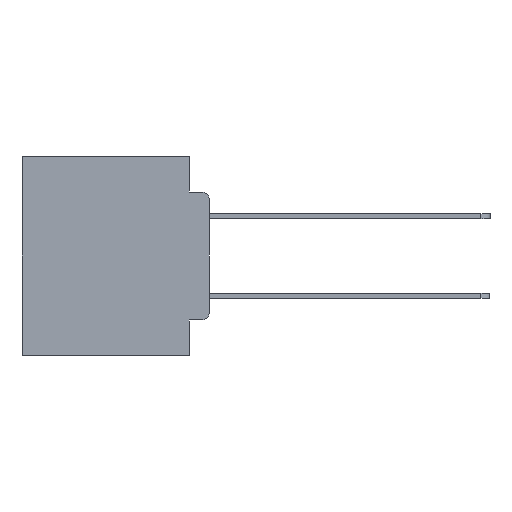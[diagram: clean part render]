
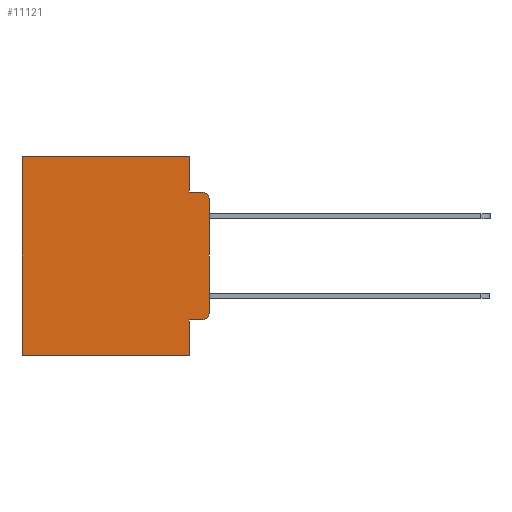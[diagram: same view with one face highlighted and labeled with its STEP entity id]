
A CAD part, left-side view. The second image highlights one B-rep face of the part: STEP entity #11121.
In plain terms, the highlighted planar face has unit normal (-1, 0, 0).
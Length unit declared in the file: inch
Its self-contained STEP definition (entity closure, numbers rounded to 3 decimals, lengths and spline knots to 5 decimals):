
#91 = EDGE_CURVE ( 'NONE', #11731, #8645, #16837, .T. ) ;
#188 = VECTOR ( 'NONE', #9509, 39.37008 ) ;
#833 = ORIENTED_EDGE ( 'NONE', *, *, #21471, .T. ) ;
#1757 = VERTEX_POINT ( 'NONE', #11568 ) ;
#2285 = ORIENTED_EDGE ( 'NONE', *, *, #91, .T. ) ;
#2340 = ORIENTED_EDGE ( 'NONE', *, *, #14090, .T. ) ;
#2466 = VERTEX_POINT ( 'NONE', #26291 ) ;
#2994 = DIRECTION ( 'NONE',  ( 0., -1., 0. ) ) ;
#3147 = VECTOR ( 'NONE', #22898, 39.37008 ) ;
#3359 = EDGE_LOOP ( 'NONE', ( #7922, #2285, #5350, #19987, #15422, #20223, #26096, #23417, #833, #2340 ) ) ;
#3412 = EDGE_CURVE ( 'NONE', #11731, #2466, #8295, .T. ) ;
#3960 = LINE ( 'NONE', #26126, #14698 ) ;
#4420 = VECTOR ( 'NONE', #9666, 39.37008 ) ;
#4872 = CARTESIAN_POINT ( 'NONE',  ( 0.298, 0.02, -0.4115 ) ) ;
#4892 = LINE ( 'NONE', #19153, #26584 ) ;
#5350 = ORIENTED_EDGE ( 'NONE', *, *, #22538, .F. ) ;
#5572 = EDGE_CURVE ( 'NONE', #7478, #25046, #7101, .T. ) ;
#6067 = CARTESIAN_POINT ( 'NONE',  ( 0.298, 0.051, 0. ) ) ;
#6334 = EDGE_CURVE ( 'NONE', #1757, #7478, #11154, .T. ) ;
#6660 = CARTESIAN_POINT ( 'NONE',  ( 0.298, 0.02, -0.1085 ) ) ;
#6828 = EDGE_CURVE ( 'NONE', #21465, #25046, #14746, .T. ) ;
#6844 = CARTESIAN_POINT ( 'NONE',  ( 0.298, 0.051, -0.5 ) ) ;
#7101 = LINE ( 'NONE', #9027, #12868 ) ;
#7158 = DIRECTION ( 'NONE',  ( 0., 0., -1. ) ) ;
#7433 = CARTESIAN_POINT ( 'NONE',  ( 0.298, 0.051, 0. ) ) ;
#7478 = VERTEX_POINT ( 'NONE', #6844 ) ;
#7873 = DIRECTION ( 'NONE',  ( 0., 1., 0. ) ) ;
#7922 = ORIENTED_EDGE ( 'NONE', *, *, #3412, .F. ) ;
#8295 = LINE ( 'NONE', #25210, #13310 ) ;
#8441 = FACE_OUTER_BOUND ( 'NONE', #3359, .T. ) ;
#8645 = VERTEX_POINT ( 'NONE', #16828 ) ;
#9027 = CARTESIAN_POINT ( 'NONE',  ( 0.298, 0., -0.5 ) ) ;
#9509 = DIRECTION ( 'NONE',  ( 0., 0., -1. ) ) ;
#9666 = DIRECTION ( 'NONE',  ( 0., 1., 0. ) ) ;
#10009 = PLANE ( 'NONE',  #25754 ) ;
#10889 = VERTEX_POINT ( 'NONE', #4872 ) ;
#10956 = DIRECTION ( 'NONE',  ( 0., -1., 0. ) ) ;
#11121 = ADVANCED_FACE ( 'NONE', ( #8441 ), #10009, .F. ) ;
#11154 = LINE ( 'NONE', #7433, #188 ) ;
#11568 = CARTESIAN_POINT ( 'NONE',  ( 0.298, 0.051, -0.4115 ) ) ;
#11731 = VERTEX_POINT ( 'NONE', #18914 ) ;
#11760 = VERTEX_POINT ( 'NONE', #13676 ) ;
#11801 = CARTESIAN_POINT ( 'NONE',  ( 0.298, 0., 0. ) ) ;
#12160 = DIRECTION ( 'NONE',  ( 1., 0., 0. ) ) ;
#12718 = VERTEX_POINT ( 'NONE', #18701 ) ;
#12868 = VECTOR ( 'NONE', #7873, 39.37008 ) ;
#12927 = CARTESIAN_POINT ( 'NONE',  ( 0.298, 0.02, -0.3915 ) ) ;
#13310 = VECTOR ( 'NONE', #25956, 39.37008 ) ;
#13333 = AXIS2_PLACEMENT_3D ( 'NONE', #6660, #20187, #7158 ) ;
#13366 = EDGE_CURVE ( 'NONE', #12718, #11760, #14624, .T. ) ;
#13676 = CARTESIAN_POINT ( 'NONE',  ( 0.298, 0.051, -0.0885 ) ) ;
#14090 = EDGE_CURVE ( 'NONE', #10889, #2466, #24205, .T. ) ;
#14343 = DIRECTION ( 'NONE',  ( 0., 0., -1. ) ) ;
#14624 = LINE ( 'NONE', #6067, #3147 ) ;
#14698 = VECTOR ( 'NONE', #2994, 39.37008 ) ;
#14746 = LINE ( 'NONE', #15899, #19580 ) ;
#15022 = DIRECTION ( 'NONE',  ( 0., 0., -1. ) ) ;
#15263 = CARTESIAN_POINT ( 'NONE',  ( 0.298, 0.473, -0.5 ) ) ;
#15422 = ORIENTED_EDGE ( 'NONE', *, *, #19486, .T. ) ;
#15899 = CARTESIAN_POINT ( 'NONE',  ( 0.298, 0.473, 0. ) ) ;
#16828 = CARTESIAN_POINT ( 'NONE',  ( 0.298, 0.02, -0.0885 ) ) ;
#16837 = CIRCLE ( 'NONE', #13333, 0.02 ) ;
#18245 = AXIS2_PLACEMENT_3D ( 'NONE', #12927, #27370, #15022 ) ;
#18701 = CARTESIAN_POINT ( 'NONE',  ( 0.298, 0.051, 0. ) ) ;
#18914 = CARTESIAN_POINT ( 'NONE',  ( 0.298, 0., -0.1085 ) ) ;
#19153 = CARTESIAN_POINT ( 'NONE',  ( 0.298, 0.051, -0.0885 ) ) ;
#19486 = EDGE_CURVE ( 'NONE', #12718, #21465, #26091, .T. ) ;
#19580 = VECTOR ( 'NONE', #14343, 39.37008 ) ;
#19987 = ORIENTED_EDGE ( 'NONE', *, *, #13366, .F. ) ;
#20187 = DIRECTION ( 'NONE',  ( -1., 0., 0. ) ) ;
#20223 = ORIENTED_EDGE ( 'NONE', *, *, #6828, .T. ) ;
#21465 = VERTEX_POINT ( 'NONE', #21995 ) ;
#21471 = EDGE_CURVE ( 'NONE', #1757, #10889, #3960, .T. ) ;
#21995 = CARTESIAN_POINT ( 'NONE',  ( 0.298, 0.473, 0. ) ) ;
#22538 = EDGE_CURVE ( 'NONE', #11760, #8645, #4892, .T. ) ;
#22898 = DIRECTION ( 'NONE',  ( 0., 0., -1. ) ) ;
#23417 = ORIENTED_EDGE ( 'NONE', *, *, #6334, .F. ) ;
#24205 = CIRCLE ( 'NONE', #18245, 0.02 ) ;
#24543 = CARTESIAN_POINT ( 'NONE',  ( 0.298, 0., 0. ) ) ;
#25046 = VERTEX_POINT ( 'NONE', #15263 ) ;
#25210 = CARTESIAN_POINT ( 'NONE',  ( 0.298, 0., 0. ) ) ;
#25754 = AXIS2_PLACEMENT_3D ( 'NONE', #24543, #12160, #26628 ) ;
#25956 = DIRECTION ( 'NONE',  ( 0., 0., -1. ) ) ;
#26091 = LINE ( 'NONE', #11801, #4420 ) ;
#26096 = ORIENTED_EDGE ( 'NONE', *, *, #5572, .F. ) ;
#26126 = CARTESIAN_POINT ( 'NONE',  ( 0.298, 0.051, -0.4115 ) ) ;
#26291 = CARTESIAN_POINT ( 'NONE',  ( 0.298, 0., -0.3915 ) ) ;
#26584 = VECTOR ( 'NONE', #10956, 39.37008 ) ;
#26628 = DIRECTION ( 'NONE',  ( 0., 0., -1. ) ) ;
#27370 = DIRECTION ( 'NONE',  ( -1., 0., 0. ) ) ;
